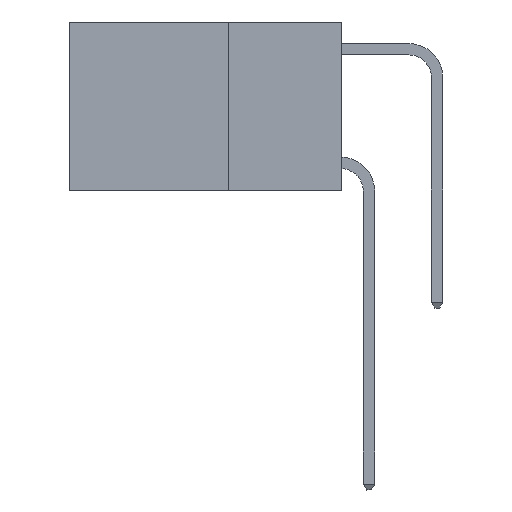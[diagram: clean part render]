
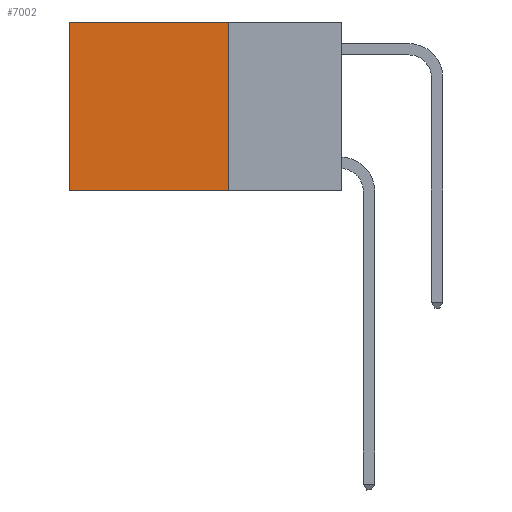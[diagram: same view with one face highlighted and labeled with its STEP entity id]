
A CAD part, left-side view. The second image highlights one B-rep face of the part: STEP entity #7002.
In plain terms, the highlighted planar face has unit normal (-1, 0, 0).
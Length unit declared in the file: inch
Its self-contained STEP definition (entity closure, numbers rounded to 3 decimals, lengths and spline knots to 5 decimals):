
#213 = VERTEX_POINT ( 'NONE', #6722 ) ;
#317 = CARTESIAN_POINT ( 'NONE',  ( 0.2625, 0.25, 0. ) ) ;
#765 = ORIENTED_EDGE ( 'NONE', *, *, #2860, .T. ) ;
#1037 = EDGE_CURVE ( 'NONE', #7708, #213, #7989, .T. ) ;
#2151 = DIRECTION ( 'NONE',  ( 0., 0., -1. ) ) ;
#2428 = VECTOR ( 'NONE', #2151, 39.37008 ) ;
#2676 = ORIENTED_EDGE ( 'NONE', *, *, #12595, .T. ) ;
#2706 = VECTOR ( 'NONE', #12761, 39.37008 ) ;
#2860 = EDGE_CURVE ( 'NONE', #14079, #19591, #22323, .T. ) ;
#3735 = EDGE_CURVE ( 'NONE', #14079, #7708, #19128, .T. ) ;
#4818 = CARTESIAN_POINT ( 'NONE',  ( 0.2625, 0.6, 0. ) ) ;
#6174 = DIRECTION ( 'NONE',  ( 0., 1., 0. ) ) ;
#6307 = DIRECTION ( 'NONE',  ( 0., 0., -1. ) ) ;
#6564 = CARTESIAN_POINT ( 'NONE',  ( 0.2625, 0.25, 0. ) ) ;
#6722 = CARTESIAN_POINT ( 'NONE',  ( 0.2625, 0.6, -0.37 ) ) ;
#7002 = ADVANCED_FACE ( 'NONE', ( #17812 ), #21330, .F. ) ;
#7708 = VERTEX_POINT ( 'NONE', #22924 ) ;
#7989 = LINE ( 'NONE', #15372, #23617 ) ;
#9266 = CARTESIAN_POINT ( 'NONE',  ( 0.2625, 0.25, 0. ) ) ;
#10155 = DIRECTION ( 'NONE',  ( 1., 0., 0. ) ) ;
#10246 = VECTOR ( 'NONE', #6307, 39.37008 ) ;
#11767 = EDGE_LOOP ( 'NONE', ( #2676, #22370, #19331, #765 ) ) ;
#12595 = EDGE_CURVE ( 'NONE', #19591, #213, #22505, .T. ) ;
#12761 = DIRECTION ( 'NONE',  ( 0., 1., 0. ) ) ;
#12885 = AXIS2_PLACEMENT_3D ( 'NONE', #19402, #10155, #13690 ) ;
#13690 = DIRECTION ( 'NONE',  ( 0., 0., -1. ) ) ;
#14079 = VERTEX_POINT ( 'NONE', #6564 ) ;
#15372 = CARTESIAN_POINT ( 'NONE',  ( 0.2625, 0.25, -0.37 ) ) ;
#17812 = FACE_OUTER_BOUND ( 'NONE', #11767, .T. ) ;
#18900 = CARTESIAN_POINT ( 'NONE',  ( 0.2625, 0.6, 0. ) ) ;
#19128 = LINE ( 'NONE', #317, #2428 ) ;
#19331 = ORIENTED_EDGE ( 'NONE', *, *, #3735, .F. ) ;
#19402 = CARTESIAN_POINT ( 'NONE',  ( 0.2625, 0.25, 0. ) ) ;
#19591 = VERTEX_POINT ( 'NONE', #4818 ) ;
#21330 = PLANE ( 'NONE',  #12885 ) ;
#22323 = LINE ( 'NONE', #9266, #2706 ) ;
#22370 = ORIENTED_EDGE ( 'NONE', *, *, #1037, .F. ) ;
#22505 = LINE ( 'NONE', #18900, #10246 ) ;
#22924 = CARTESIAN_POINT ( 'NONE',  ( 0.2625, 0.25, -0.37 ) ) ;
#23617 = VECTOR ( 'NONE', #6174, 39.37008 ) ;
